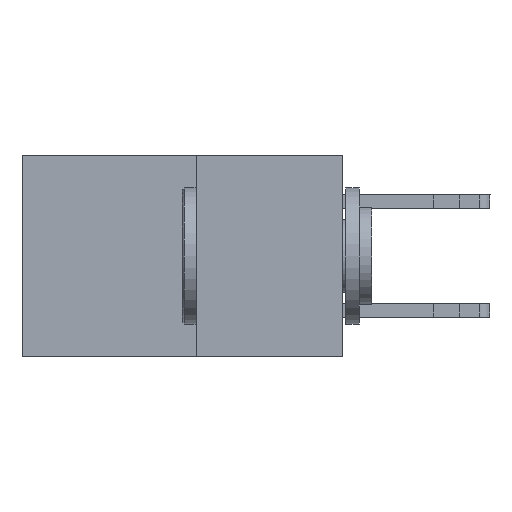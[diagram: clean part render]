
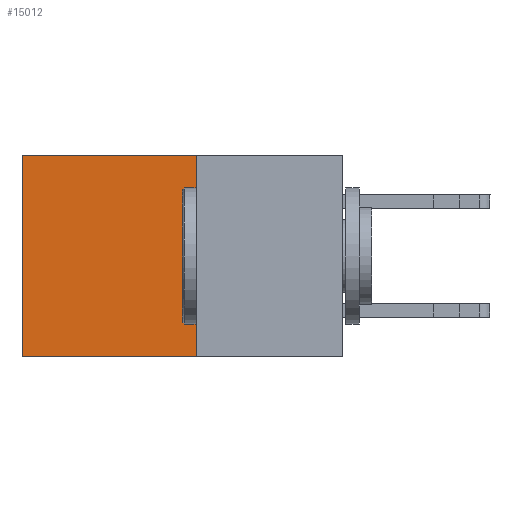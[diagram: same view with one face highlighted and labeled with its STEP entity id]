
A CAD part, left-side view. The second image highlights one B-rep face of the part: STEP entity #15012.
In plain terms, the highlighted planar face has unit normal (-1, 0, 0).
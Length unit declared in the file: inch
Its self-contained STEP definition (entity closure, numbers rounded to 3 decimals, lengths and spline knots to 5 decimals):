
#416 = VERTEX_POINT ( 'NONE', #7692 ) ;
#623 = VECTOR ( 'NONE', #21998, 39.37008 ) ;
#1937 = LINE ( 'NONE', #9812, #20776 ) ;
#2399 = VERTEX_POINT ( 'NONE', #11380 ) ;
#2623 = EDGE_CURVE ( 'NONE', #14998, #6371, #1937, .T. ) ;
#3201 = CARTESIAN_POINT ( 'NONE',  ( 0.277, 0.59, 0. ) ) ;
#3630 = EDGE_CURVE ( 'NONE', #6371, #2399, #16348, .T. ) ;
#4325 = ORIENTED_EDGE ( 'NONE', *, *, #15370, .F. ) ;
#4767 = DIRECTION ( 'NONE',  ( 0., 0., -1. ) ) ;
#5010 = VECTOR ( 'NONE', #11524, 39.37008 ) ;
#5152 = CARTESIAN_POINT ( 'NONE',  ( 0.277, 0.27, -0.37 ) ) ;
#5930 = DIRECTION ( 'NONE',  ( 0., 1., 0. ) ) ;
#6371 = VERTEX_POINT ( 'NONE', #3201 ) ;
#6705 = EDGE_LOOP ( 'NONE', ( #17745, #4325, #8712, #11226 ) ) ;
#7692 = CARTESIAN_POINT ( 'NONE',  ( 0.277, 0.27, -0.37 ) ) ;
#8712 = ORIENTED_EDGE ( 'NONE', *, *, #23544, .F. ) ;
#9582 = CARTESIAN_POINT ( 'NONE',  ( 0.277, 0.27, -0.37 ) ) ;
#9812 = CARTESIAN_POINT ( 'NONE',  ( 0.277, 0.27, 0. ) ) ;
#10158 = VECTOR ( 'NONE', #12252, 39.37008 ) ;
#11226 = ORIENTED_EDGE ( 'NONE', *, *, #2623, .T. ) ;
#11380 = CARTESIAN_POINT ( 'NONE',  ( 0.277, 0.59, -0.37 ) ) ;
#11524 = DIRECTION ( 'NONE',  ( 0., 0., -1. ) ) ;
#12252 = DIRECTION ( 'NONE',  ( 0., 1., 0. ) ) ;
#13930 = CARTESIAN_POINT ( 'NONE',  ( 0.277, 0.27, -0.37 ) ) ;
#14043 = LINE ( 'NONE', #13930, #10158 ) ;
#14702 = FACE_OUTER_BOUND ( 'NONE', #6705, .T. ) ;
#14818 = PLANE ( 'NONE',  #18388 ) ;
#14998 = VERTEX_POINT ( 'NONE', #16018 ) ;
#15012 = ADVANCED_FACE ( 'NONE', ( #14702 ), #14818, .F. ) ;
#15370 = EDGE_CURVE ( 'NONE', #416, #2399, #14043, .T. ) ;
#16018 = CARTESIAN_POINT ( 'NONE',  ( 0.277, 0.27, 0. ) ) ;
#16078 = CARTESIAN_POINT ( 'NONE',  ( 0.277, 0.59, -0.37 ) ) ;
#16348 = LINE ( 'NONE', #16078, #623 ) ;
#16881 = DIRECTION ( 'NONE',  ( 1., 0., 0. ) ) ;
#17208 = LINE ( 'NONE', #9582, #5010 ) ;
#17745 = ORIENTED_EDGE ( 'NONE', *, *, #3630, .T. ) ;
#18388 = AXIS2_PLACEMENT_3D ( 'NONE', #5152, #16881, #4767 ) ;
#20776 = VECTOR ( 'NONE', #5930, 39.37008 ) ;
#21998 = DIRECTION ( 'NONE',  ( 0., 0., -1. ) ) ;
#23544 = EDGE_CURVE ( 'NONE', #14998, #416, #17208, .T. ) ;
